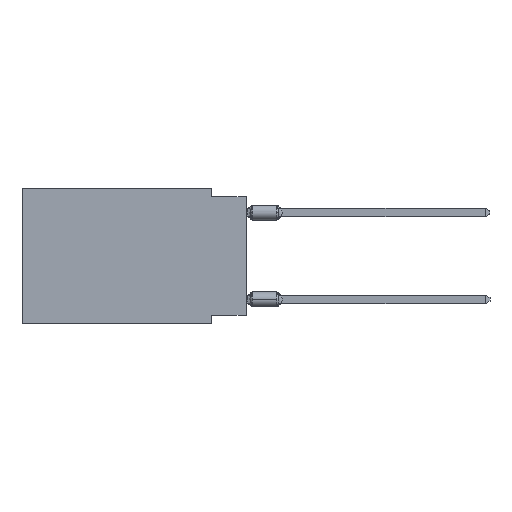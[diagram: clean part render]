
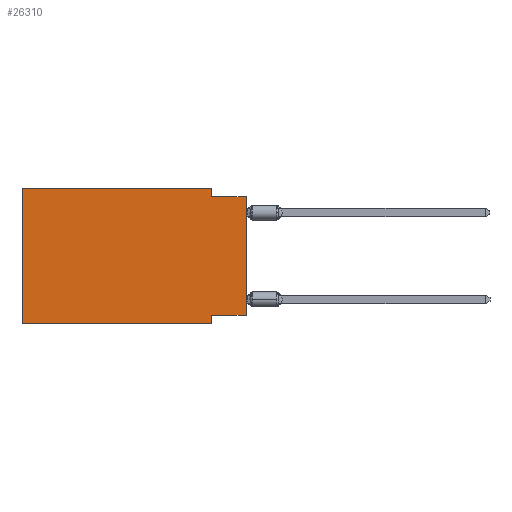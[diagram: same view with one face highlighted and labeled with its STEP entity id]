
A CAD part, left-side view. The second image highlights one B-rep face of the part: STEP entity #26310.
In plain terms, the highlighted planar face has unit normal (-1, 0, 0).
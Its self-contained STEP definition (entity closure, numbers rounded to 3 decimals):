
#95 = EDGE_CURVE ( 'NONE', #15796, #9065, #6558, .T. ) ;
#116 = VECTOR ( 'NONE', #11298, 1000. ) ;
#268 = VERTEX_POINT ( 'NONE', #4920 ) ;
#288 = PLANE ( 'NONE',  #2918 ) ;
#628 = LINE ( 'NONE', #25179, #18299 ) ;
#908 = VERTEX_POINT ( 'NONE', #10723 ) ;
#1254 = ORIENTED_EDGE ( 'NONE', *, *, #17388, .F. ) ;
#1764 = ORIENTED_EDGE ( 'NONE', *, *, #2903, .T. ) ;
#2837 = CARTESIAN_POINT ( 'NONE',  ( 0., 2.54, 0. ) ) ;
#2903 = EDGE_CURVE ( 'NONE', #8940, #908, #16015, .T. ) ;
#2918 = AXIS2_PLACEMENT_3D ( 'NONE', #17060, #16922, #4901 ) ;
#3111 = EDGE_CURVE ( 'NONE', #9065, #15910, #15685, .T. ) ;
#3394 = CARTESIAN_POINT ( 'NONE',  ( 0., 0., -9.271 ) ) ;
#3614 = ORIENTED_EDGE ( 'NONE', *, *, #21277, .F. ) ;
#3800 = CARTESIAN_POINT ( 'NONE',  ( 0., 16.383, 0. ) ) ;
#3805 = CARTESIAN_POINT ( 'NONE',  ( 0., 0., -9.271 ) ) ;
#4838 = DIRECTION ( 'NONE',  ( 0., 0., -1. ) ) ;
#4901 = DIRECTION ( 'NONE',  ( 0., 0., -1. ) ) ;
#4920 = CARTESIAN_POINT ( 'NONE',  ( 0., 2.54, -9.906 ) ) ;
#5187 = VERTEX_POINT ( 'NONE', #18475 ) ;
#6366 = VECTOR ( 'NONE', #14234, 1000. ) ;
#6558 = LINE ( 'NONE', #15172, #8866 ) ;
#7843 = VECTOR ( 'NONE', #16960, 1000. ) ;
#8025 = DIRECTION ( 'NONE',  ( 0., 1., 0. ) ) ;
#8285 = LINE ( 'NONE', #3800, #15340 ) ;
#8435 = CARTESIAN_POINT ( 'NONE',  ( 0., 2.54, -9.271 ) ) ;
#8561 = VECTOR ( 'NONE', #15272, 1000. ) ;
#8866 = VECTOR ( 'NONE', #15308, 1000. ) ;
#8940 = VERTEX_POINT ( 'NONE', #3805 ) ;
#9065 = VERTEX_POINT ( 'NONE', #2837 ) ;
#10723 = CARTESIAN_POINT ( 'NONE',  ( 0., 0., -0.635 ) ) ;
#10945 = CARTESIAN_POINT ( 'NONE',  ( 0., 16.383, -9.906 ) ) ;
#11016 = ORIENTED_EDGE ( 'NONE', *, *, #13708, .F. ) ;
#11298 = DIRECTION ( 'NONE',  ( 0., -1., 0. ) ) ;
#11730 = EDGE_CURVE ( 'NONE', #15910, #908, #18128, .T. ) ;
#11881 = CARTESIAN_POINT ( 'NONE',  ( 0., 16.383, 0. ) ) ;
#12460 = ORIENTED_EDGE ( 'NONE', *, *, #95, .F. ) ;
#13624 = CARTESIAN_POINT ( 'NONE',  ( 0., 2.54, 0. ) ) ;
#13708 = EDGE_CURVE ( 'NONE', #23150, #268, #628, .T. ) ;
#14226 = EDGE_CURVE ( 'NONE', #5187, #268, #23239, .T. ) ;
#14234 = DIRECTION ( 'NONE',  ( 0., 0., 1. ) ) ;
#14343 = VECTOR ( 'NONE', #8025, 1000. ) ;
#14345 = ORIENTED_EDGE ( 'NONE', *, *, #3111, .F. ) ;
#15083 = ORIENTED_EDGE ( 'NONE', *, *, #14226, .T. ) ;
#15172 = CARTESIAN_POINT ( 'NONE',  ( 0., 16.383, 0. ) ) ;
#15272 = DIRECTION ( 'NONE',  ( 0., 0., -1. ) ) ;
#15308 = DIRECTION ( 'NONE',  ( 0., -1., 0. ) ) ;
#15340 = VECTOR ( 'NONE', #20988, 1000. ) ;
#15685 = LINE ( 'NONE', #13624, #8561 ) ;
#15796 = VERTEX_POINT ( 'NONE', #11881 ) ;
#15910 = VERTEX_POINT ( 'NONE', #21023 ) ;
#15962 = ORIENTED_EDGE ( 'NONE', *, *, #11730, .F. ) ;
#16015 = LINE ( 'NONE', #18067, #6366 ) ;
#16922 = DIRECTION ( 'NONE',  ( 1., 0., 0. ) ) ;
#16960 = DIRECTION ( 'NONE',  ( 0., -1., 0. ) ) ;
#17060 = CARTESIAN_POINT ( 'NONE',  ( 0., 16.383, 0. ) ) ;
#17388 = EDGE_CURVE ( 'NONE', #8940, #23150, #26336, .T. ) ;
#18067 = CARTESIAN_POINT ( 'NONE',  ( 0., 0., 0. ) ) ;
#18128 = LINE ( 'NONE', #24132, #116 ) ;
#18299 = VECTOR ( 'NONE', #4838, 1000. ) ;
#18475 = CARTESIAN_POINT ( 'NONE',  ( 0., 16.383, -9.906 ) ) ;
#20988 = DIRECTION ( 'NONE',  ( 0., 0., 1. ) ) ;
#21023 = CARTESIAN_POINT ( 'NONE',  ( 0., 2.54, -0.635 ) ) ;
#21277 = EDGE_CURVE ( 'NONE', #5187, #15796, #8285, .T. ) ;
#22559 = EDGE_LOOP ( 'NONE', ( #1764, #15962, #14345, #12460, #3614, #15083, #11016, #1254 ) ) ;
#23150 = VERTEX_POINT ( 'NONE', #8435 ) ;
#23239 = LINE ( 'NONE', #10945, #7843 ) ;
#23603 = FACE_OUTER_BOUND ( 'NONE', #22559, .T. ) ;
#24132 = CARTESIAN_POINT ( 'NONE',  ( 0., 0., -0.635 ) ) ;
#25179 = CARTESIAN_POINT ( 'NONE',  ( 0., 2.54, -9.906 ) ) ;
#26310 = ADVANCED_FACE ( 'NONE', ( #23603 ), #288, .F. ) ;
#26336 = LINE ( 'NONE', #3394, #14343 ) ;
